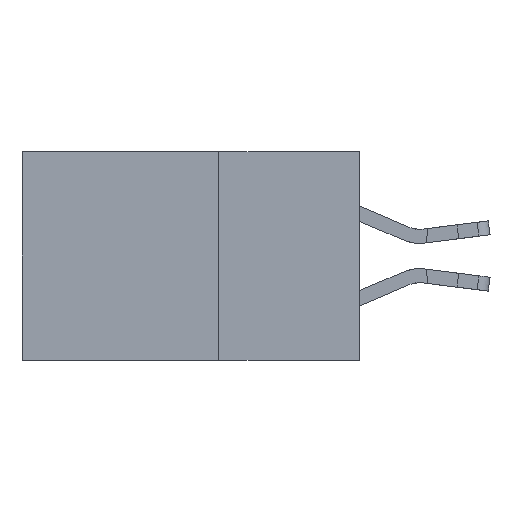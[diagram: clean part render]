
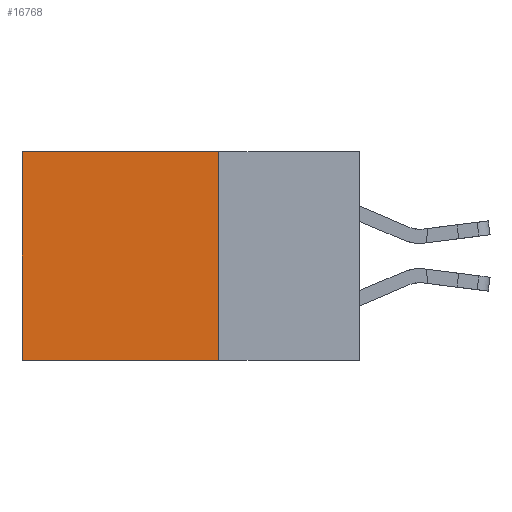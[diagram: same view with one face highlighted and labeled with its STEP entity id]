
A CAD part, left-side view. The second image highlights one B-rep face of the part: STEP entity #16768.
In plain terms, the highlighted planar face has unit normal (-1, 0, 0).
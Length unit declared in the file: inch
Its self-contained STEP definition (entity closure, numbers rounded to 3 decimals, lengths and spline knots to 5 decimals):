
#618 = CARTESIAN_POINT ( 'NONE',  ( 0.2875, 0.25, 0. ) ) ;
#1048 = DIRECTION ( 'NONE',  ( 0., 1., 0. ) ) ;
#2061 = CARTESIAN_POINT ( 'NONE',  ( 0.2875, 0.25, 0. ) ) ;
#2595 = CARTESIAN_POINT ( 'NONE',  ( 0.2875, 0.25, -0.37 ) ) ;
#3714 = EDGE_CURVE ( 'NONE', #16484, #22370, #11224, .T. ) ;
#4525 = LINE ( 'NONE', #12712, #17021 ) ;
#4528 = EDGE_CURVE ( 'NONE', #15132, #16484, #4525, .T. ) ;
#5181 = CARTESIAN_POINT ( 'NONE',  ( 0.2875, 0.6, 0. ) ) ;
#5505 = DIRECTION ( 'NONE',  ( 1., 0., 0. ) ) ;
#5560 = CARTESIAN_POINT ( 'NONE',  ( 0.2875, 0.6, -0.37 ) ) ;
#6215 = EDGE_CURVE ( 'NONE', #15132, #16857, #11439, .T. ) ;
#6873 = VECTOR ( 'NONE', #1048, 39.37008 ) ;
#7064 = EDGE_CURVE ( 'NONE', #16857, #22370, #16941, .T. ) ;
#7151 = ORIENTED_EDGE ( 'NONE', *, *, #6215, .T. ) ;
#7170 = DIRECTION ( 'NONE',  ( 0., 0., -1. ) ) ;
#8642 = ORIENTED_EDGE ( 'NONE', *, *, #7064, .T. ) ;
#9367 = VECTOR ( 'NONE', #12326, 39.37008 ) ;
#10004 = DIRECTION ( 'NONE',  ( 0., 1., 0. ) ) ;
#11224 = LINE ( 'NONE', #19571, #6873 ) ;
#11439 = LINE ( 'NONE', #2061, #18436 ) ;
#12326 = DIRECTION ( 'NONE',  ( 0., 0., -1. ) ) ;
#12712 = CARTESIAN_POINT ( 'NONE',  ( 0.2875, 0.25, 0. ) ) ;
#14851 = PLANE ( 'NONE',  #22843 ) ;
#15132 = VERTEX_POINT ( 'NONE', #618 ) ;
#16267 = EDGE_LOOP ( 'NONE', ( #8642, #21175, #17715, #7151 ) ) ;
#16484 = VERTEX_POINT ( 'NONE', #2595 ) ;
#16768 = ADVANCED_FACE ( 'NONE', ( #22441 ), #14851, .F. ) ;
#16857 = VERTEX_POINT ( 'NONE', #5181 ) ;
#16941 = LINE ( 'NONE', #19707, #9367 ) ;
#17021 = VECTOR ( 'NONE', #7170, 39.37008 ) ;
#17715 = ORIENTED_EDGE ( 'NONE', *, *, #4528, .F. ) ;
#18436 = VECTOR ( 'NONE', #10004, 39.37008 ) ;
#19571 = CARTESIAN_POINT ( 'NONE',  ( 0.2875, 0.25, -0.37 ) ) ;
#19707 = CARTESIAN_POINT ( 'NONE',  ( 0.2875, 0.6, 0. ) ) ;
#20042 = DIRECTION ( 'NONE',  ( 0., 0., -1. ) ) ;
#21175 = ORIENTED_EDGE ( 'NONE', *, *, #3714, .F. ) ;
#22370 = VERTEX_POINT ( 'NONE', #5560 ) ;
#22441 = FACE_OUTER_BOUND ( 'NONE', #16267, .T. ) ;
#22843 = AXIS2_PLACEMENT_3D ( 'NONE', #23957, #5505, #20042 ) ;
#23957 = CARTESIAN_POINT ( 'NONE',  ( 0.2875, 0.25, 0. ) ) ;
